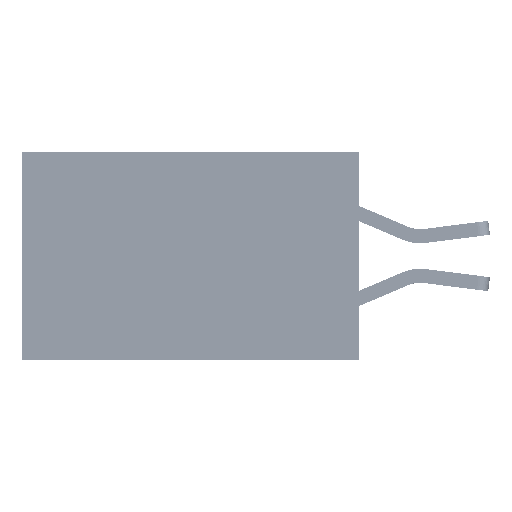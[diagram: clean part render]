
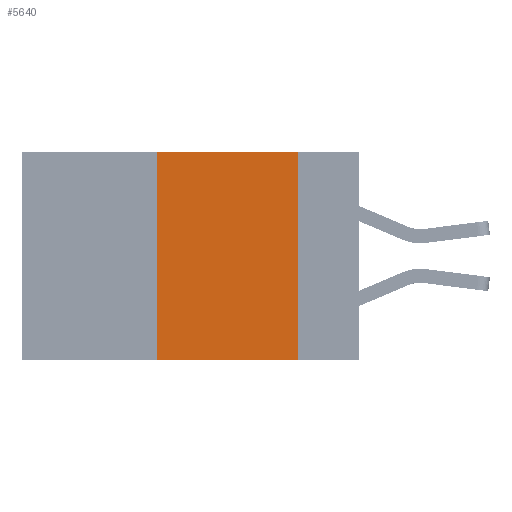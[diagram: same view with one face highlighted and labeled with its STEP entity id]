
A CAD part, left-side view. The second image highlights one B-rep face of the part: STEP entity #5640.
In plain terms, the highlighted planar face has unit normal (-1, 0, 0).
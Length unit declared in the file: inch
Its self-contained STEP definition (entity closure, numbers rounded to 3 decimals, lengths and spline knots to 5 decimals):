
#115 = LINE ( 'NONE', #26100, #28850 ) ;
#1045 = VECTOR ( 'NONE', #48399, 39.37008 ) ;
#2049 = ORIENTED_EDGE ( 'NONE', *, *, #36837, .F. ) ;
#2290 = LINE ( 'NONE', #9733, #1045 ) ;
#4551 = CARTESIAN_POINT ( 'NONE',  ( 0., 0.36, -0.37 ) ) ;
#4757 = EDGE_CURVE ( 'NONE', #26144, #31894, #29217, .T. ) ;
#5640 = ADVANCED_FACE ( 'NONE', ( #31538 ), #15419, .F. ) ;
#6034 = EDGE_LOOP ( 'NONE', ( #49882, #2049, #32018, #17924 ) ) ;
#7533 = CARTESIAN_POINT ( 'NONE',  ( 0., 0.6, 0. ) ) ;
#9733 = CARTESIAN_POINT ( 'NONE',  ( 0., 0.6, 0. ) ) ;
#10133 = CARTESIAN_POINT ( 'NONE',  ( 0., 0.11, -0.37 ) ) ;
#10382 = CARTESIAN_POINT ( 'NONE',  ( 0., 0.11, 0. ) ) ;
#13804 = EDGE_CURVE ( 'NONE', #45757, #20668, #115, .T. ) ;
#14343 = DIRECTION ( 'NONE',  ( 0., 0., -1. ) ) ;
#15419 = PLANE ( 'NONE',  #49307 ) ;
#17924 = ORIENTED_EDGE ( 'NONE', *, *, #47411, .T. ) ;
#17969 = VECTOR ( 'NONE', #23546, 39.37008 ) ;
#18870 = VECTOR ( 'NONE', #14343, 39.37008 ) ;
#19340 = DIRECTION ( 'NONE',  ( 0., 0., -1. ) ) ;
#20668 = VERTEX_POINT ( 'NONE', #28037 ) ;
#23546 = DIRECTION ( 'NONE',  ( 0., -1., 0. ) ) ;
#26100 = CARTESIAN_POINT ( 'NONE',  ( 0., 0.36, 0. ) ) ;
#26144 = VERTEX_POINT ( 'NONE', #29836 ) ;
#28037 = CARTESIAN_POINT ( 'NONE',  ( 0., 0.36, 0. ) ) ;
#28310 = LINE ( 'NONE', #42806, #17969 ) ;
#28850 = VECTOR ( 'NONE', #37771, 39.37008 ) ;
#29217 = LINE ( 'NONE', #10382, #18870 ) ;
#29836 = CARTESIAN_POINT ( 'NONE',  ( 0., 0.11, 0. ) ) ;
#31538 = FACE_OUTER_BOUND ( 'NONE', #6034, .T. ) ;
#31894 = VERTEX_POINT ( 'NONE', #10133 ) ;
#32018 = ORIENTED_EDGE ( 'NONE', *, *, #13804, .F. ) ;
#36837 = EDGE_CURVE ( 'NONE', #20668, #26144, #2290, .T. ) ;
#37771 = DIRECTION ( 'NONE',  ( 0., 0., 1. ) ) ;
#42523 = DIRECTION ( 'NONE',  ( 1., 0., 0. ) ) ;
#42806 = CARTESIAN_POINT ( 'NONE',  ( 0., 0.6, -0.37 ) ) ;
#45757 = VERTEX_POINT ( 'NONE', #4551 ) ;
#47411 = EDGE_CURVE ( 'NONE', #45757, #31894, #28310, .T. ) ;
#48399 = DIRECTION ( 'NONE',  ( 0., -1., 0. ) ) ;
#49307 = AXIS2_PLACEMENT_3D ( 'NONE', #7533, #42523, #19340 ) ;
#49882 = ORIENTED_EDGE ( 'NONE', *, *, #4757, .F. ) ;
